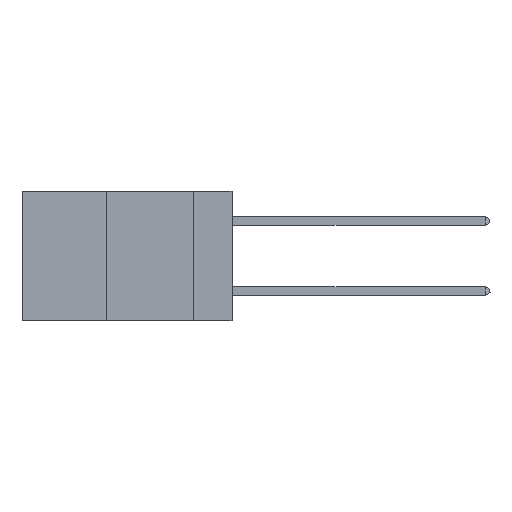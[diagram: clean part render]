
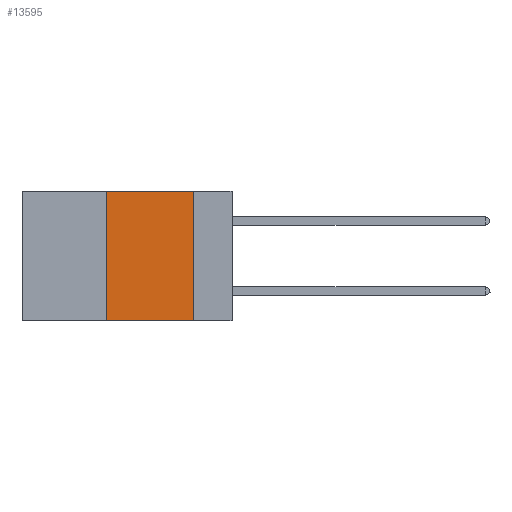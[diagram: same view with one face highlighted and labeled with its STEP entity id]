
A CAD part, left-side view. The second image highlights one B-rep face of the part: STEP entity #13595.
In plain terms, the highlighted planar face has unit normal (-1, 0, 0).
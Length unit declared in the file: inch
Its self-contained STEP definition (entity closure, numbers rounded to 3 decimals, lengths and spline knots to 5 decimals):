
#622 = VECTOR ( 'NONE', #9112, 39.37008 ) ;
#956 = EDGE_CURVE ( 'NONE', #23520, #9383, #6969, .T. ) ;
#1312 = CARTESIAN_POINT ( 'NONE',  ( 0., 0.6, -0.37 ) ) ;
#1813 = DIRECTION ( 'NONE',  ( 0., 0., -1. ) ) ;
#3661 = CARTESIAN_POINT ( 'NONE',  ( 0., 0.36, -0.37 ) ) ;
#4077 = LINE ( 'NONE', #21312, #20020 ) ;
#4466 = CARTESIAN_POINT ( 'NONE',  ( 0., 0.36, 0. ) ) ;
#5957 = CARTESIAN_POINT ( 'NONE',  ( 0., 0.11, 0. ) ) ;
#6969 = LINE ( 'NONE', #25441, #622 ) ;
#9112 = DIRECTION ( 'NONE',  ( 0., -1., 0. ) ) ;
#9143 = EDGE_LOOP ( 'NONE', ( #12564, #22587, #13519, #12570 ) ) ;
#9383 = VERTEX_POINT ( 'NONE', #21457 ) ;
#10229 = EDGE_CURVE ( 'NONE', #9383, #12754, #11252, .T. ) ;
#10248 = VERTEX_POINT ( 'NONE', #3661 ) ;
#11252 = LINE ( 'NONE', #5957, #26272 ) ;
#12432 = LINE ( 'NONE', #1312, #24586 ) ;
#12564 = ORIENTED_EDGE ( 'NONE', *, *, #10229, .F. ) ;
#12570 = ORIENTED_EDGE ( 'NONE', *, *, #12821, .T. ) ;
#12754 = VERTEX_POINT ( 'NONE', #19761 ) ;
#12821 = EDGE_CURVE ( 'NONE', #10248, #12754, #12432, .T. ) ;
#13181 = DIRECTION ( 'NONE',  ( 0., 0., 1. ) ) ;
#13519 = ORIENTED_EDGE ( 'NONE', *, *, #21769, .F. ) ;
#13595 = ADVANCED_FACE ( 'NONE', ( #24206 ), #22135, .F. ) ;
#16045 = CARTESIAN_POINT ( 'NONE',  ( 0., 0.6, 0. ) ) ;
#16131 = DIRECTION ( 'NONE',  ( 1., 0., 0. ) ) ;
#19663 = DIRECTION ( 'NONE',  ( 0., -1., 0. ) ) ;
#19761 = CARTESIAN_POINT ( 'NONE',  ( 0., 0.11, -0.37 ) ) ;
#20020 = VECTOR ( 'NONE', #13181, 39.37008 ) ;
#20979 = AXIS2_PLACEMENT_3D ( 'NONE', #16045, #16131, #1813 ) ;
#21312 = CARTESIAN_POINT ( 'NONE',  ( 0., 0.36, 0. ) ) ;
#21457 = CARTESIAN_POINT ( 'NONE',  ( 0., 0.11, 0. ) ) ;
#21769 = EDGE_CURVE ( 'NONE', #10248, #23520, #4077, .T. ) ;
#22039 = DIRECTION ( 'NONE',  ( 0., 0., -1. ) ) ;
#22135 = PLANE ( 'NONE',  #20979 ) ;
#22587 = ORIENTED_EDGE ( 'NONE', *, *, #956, .F. ) ;
#23520 = VERTEX_POINT ( 'NONE', #4466 ) ;
#24206 = FACE_OUTER_BOUND ( 'NONE', #9143, .T. ) ;
#24586 = VECTOR ( 'NONE', #19663, 39.37008 ) ;
#25441 = CARTESIAN_POINT ( 'NONE',  ( 0., 0.6, 0. ) ) ;
#26272 = VECTOR ( 'NONE', #22039, 39.37008 ) ;
